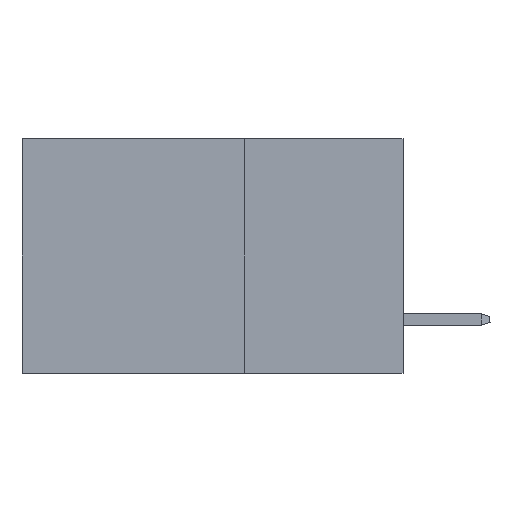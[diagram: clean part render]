
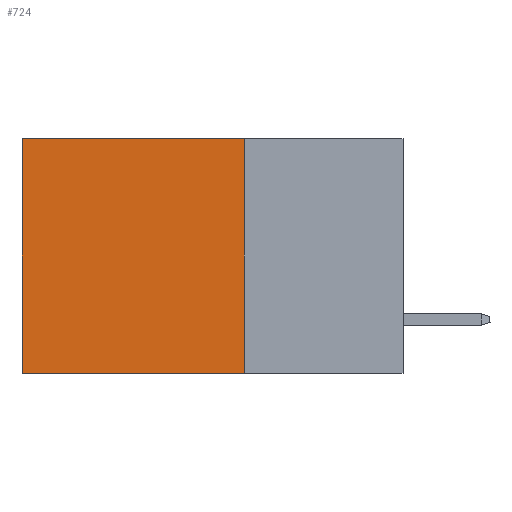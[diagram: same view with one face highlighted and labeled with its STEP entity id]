
A CAD part, left-side view. The second image highlights one B-rep face of the part: STEP entity #724.
In plain terms, the highlighted planar face has unit normal (-1, 0, 0).
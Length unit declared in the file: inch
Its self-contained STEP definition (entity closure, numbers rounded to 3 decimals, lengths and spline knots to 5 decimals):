
#114 = CARTESIAN_POINT ( 'NONE',  ( 0.2875, 0.25, -0.37 ) ) ;
#394 = ORIENTED_EDGE ( 'NONE', *, *, #20033, .T. ) ;
#724 = ADVANCED_FACE ( 'NONE', ( #9006 ), #23342, .F. ) ;
#2070 = VECTOR ( 'NONE', #23497, 39.37008 ) ;
#2556 = CARTESIAN_POINT ( 'NONE',  ( 0.2875, 0.6, 0. ) ) ;
#3394 = CARTESIAN_POINT ( 'NONE',  ( 0.2875, 0.6, -0.37 ) ) ;
#4451 = VECTOR ( 'NONE', #15122, 39.37008 ) ;
#5185 = CARTESIAN_POINT ( 'NONE',  ( 0.2875, 0.25, 0. ) ) ;
#5641 = DIRECTION ( 'NONE',  ( 0., 0., -1. ) ) ;
#6095 = CARTESIAN_POINT ( 'NONE',  ( 0.2875, 0.25, 0. ) ) ;
#6220 = VERTEX_POINT ( 'NONE', #2556 ) ;
#7368 = EDGE_CURVE ( 'NONE', #12846, #18959, #8930, .T. ) ;
#7762 = EDGE_CURVE ( 'NONE', #6220, #18959, #14467, .T. ) ;
#8578 = CARTESIAN_POINT ( 'NONE',  ( 0.2875, 0.25, -0.37 ) ) ;
#8930 = LINE ( 'NONE', #8578, #2070 ) ;
#8940 = CARTESIAN_POINT ( 'NONE',  ( 0.2875, 0.25, 0. ) ) ;
#8963 = LINE ( 'NONE', #12660, #9140 ) ;
#9006 = FACE_OUTER_BOUND ( 'NONE', #19740, .T. ) ;
#9140 = VECTOR ( 'NONE', #10633, 39.37008 ) ;
#9269 = AXIS2_PLACEMENT_3D ( 'NONE', #5185, #21666, #12361 ) ;
#10215 = ORIENTED_EDGE ( 'NONE', *, *, #7368, .F. ) ;
#10633 = DIRECTION ( 'NONE',  ( 0., 0., -1. ) ) ;
#10656 = ORIENTED_EDGE ( 'NONE', *, *, #11012, .F. ) ;
#10722 = LINE ( 'NONE', #8940, #4451 ) ;
#11012 = EDGE_CURVE ( 'NONE', #11176, #12846, #8963, .T. ) ;
#11176 = VERTEX_POINT ( 'NONE', #6095 ) ;
#12361 = DIRECTION ( 'NONE',  ( 0., 0., -1. ) ) ;
#12660 = CARTESIAN_POINT ( 'NONE',  ( 0.2875, 0.25, 0. ) ) ;
#12807 = CARTESIAN_POINT ( 'NONE',  ( 0.2875, 0.6, 0. ) ) ;
#12846 = VERTEX_POINT ( 'NONE', #114 ) ;
#12995 = ORIENTED_EDGE ( 'NONE', *, *, #7762, .T. ) ;
#14467 = LINE ( 'NONE', #12807, #20392 ) ;
#15122 = DIRECTION ( 'NONE',  ( 0., 1., 0. ) ) ;
#18959 = VERTEX_POINT ( 'NONE', #3394 ) ;
#19740 = EDGE_LOOP ( 'NONE', ( #12995, #10215, #10656, #394 ) ) ;
#20033 = EDGE_CURVE ( 'NONE', #11176, #6220, #10722, .T. ) ;
#20392 = VECTOR ( 'NONE', #5641, 39.37008 ) ;
#21666 = DIRECTION ( 'NONE',  ( 1., 0., 0. ) ) ;
#23342 = PLANE ( 'NONE',  #9269 ) ;
#23497 = DIRECTION ( 'NONE',  ( 0., 1., 0. ) ) ;
